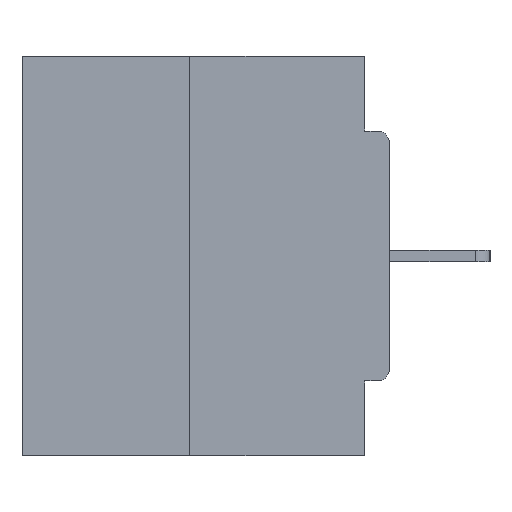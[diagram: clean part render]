
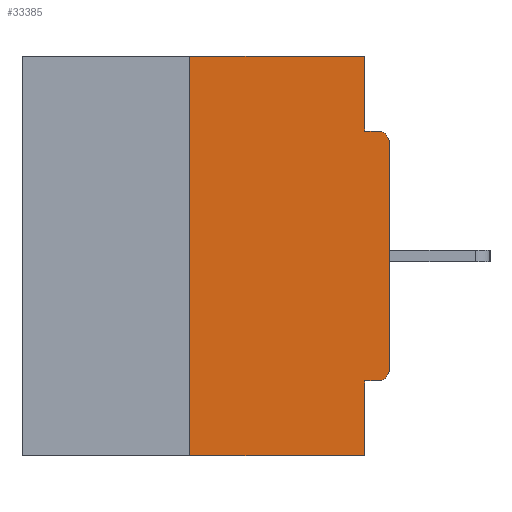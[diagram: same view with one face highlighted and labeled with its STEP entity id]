
A CAD part, left-side view. The second image highlights one B-rep face of the part: STEP entity #33385.
In plain terms, the highlighted planar face has unit normal (-1, 0, 0).
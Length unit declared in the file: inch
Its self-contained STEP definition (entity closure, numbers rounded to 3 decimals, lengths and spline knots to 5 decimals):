
#1274 = VERTEX_POINT ( 'NONE', #31369 ) ;
#2604 = CARTESIAN_POINT ( 'NONE',  ( 0., 0., -0.0935 ) ) ;
#3600 = AXIS2_PLACEMENT_3D ( 'NONE', #32483, #29717, #26374 ) ;
#3824 = VERTEX_POINT ( 'NONE', #5330 ) ;
#4188 = AXIS2_PLACEMENT_3D ( 'NONE', #30017, #5904, #33149 ) ;
#5330 = CARTESIAN_POINT ( 'NONE',  ( 0., 0.031, -0.4065 ) ) ;
#5664 = VECTOR ( 'NONE', #18033, 39.37008 ) ;
#5861 = CARTESIAN_POINT ( 'NONE',  ( 0., 0., -0.3915 ) ) ;
#5904 = DIRECTION ( 'NONE',  ( -1., 0., 0. ) ) ;
#6030 = ORIENTED_EDGE ( 'NONE', *, *, #16858, .F. ) ;
#6788 = CARTESIAN_POINT ( 'NONE',  ( 0., 0.031, -0.5 ) ) ;
#7313 = DIRECTION ( 'NONE',  ( 0., -1., 0. ) ) ;
#7596 = CARTESIAN_POINT ( 'NONE',  ( 0., 0.46, -0.5 ) ) ;
#7690 = DIRECTION ( 'NONE',  ( 0., 0., -1. ) ) ;
#7741 = AXIS2_PLACEMENT_3D ( 'NONE', #16851, #10987, #31230 ) ;
#10088 = VERTEX_POINT ( 'NONE', #12176 ) ;
#10491 = CARTESIAN_POINT ( 'NONE',  ( 0., 0.015, -0.0935 ) ) ;
#10602 = VERTEX_POINT ( 'NONE', #5861 ) ;
#10753 = DIRECTION ( 'NONE',  ( 0., 1., 0. ) ) ;
#10987 = DIRECTION ( 'NONE',  ( 1., 0., 0. ) ) ;
#11127 = EDGE_CURVE ( 'NONE', #16097, #1274, #31226, .T. ) ;
#11140 = CIRCLE ( 'NONE', #3600, 0.015 ) ;
#12176 = CARTESIAN_POINT ( 'NONE',  ( 0., 0.25, 0. ) ) ;
#13033 = DIRECTION ( 'NONE',  ( 0., 0., 1. ) ) ;
#13293 = CARTESIAN_POINT ( 'NONE',  ( 0., 0.015, -0.4065 ) ) ;
#13411 = VECTOR ( 'NONE', #29967, 39.37008 ) ;
#13440 = CARTESIAN_POINT ( 'NONE',  ( 0., 0., -0.1085 ) ) ;
#15806 = ORIENTED_EDGE ( 'NONE', *, *, #22872, .T. ) ;
#16097 = VERTEX_POINT ( 'NONE', #23859 ) ;
#16159 = LINE ( 'NONE', #19076, #30032 ) ;
#16303 = VERTEX_POINT ( 'NONE', #6788 ) ;
#16851 = CARTESIAN_POINT ( 'NONE',  ( 0., 0.46, 0. ) ) ;
#16858 = EDGE_CURVE ( 'NONE', #10088, #16097, #27702, .T. ) ;
#17041 = PLANE ( 'NONE',  #7741 ) ;
#17614 = CARTESIAN_POINT ( 'NONE',  ( 0., 0.031, -0.5 ) ) ;
#18033 = DIRECTION ( 'NONE',  ( 0., -1., 0. ) ) ;
#18091 = VECTOR ( 'NONE', #7690, 39.37008 ) ;
#19032 = VECTOR ( 'NONE', #10753, 39.37008 ) ;
#19076 = CARTESIAN_POINT ( 'NONE',  ( 0., 0.25, 0. ) ) ;
#19533 = DIRECTION ( 'NONE',  ( 0., -1., 0. ) ) ;
#19985 = EDGE_CURVE ( 'NONE', #21564, #10088, #16159, .T. ) ;
#20447 = ORIENTED_EDGE ( 'NONE', *, *, #33771, .F. ) ;
#21071 = CIRCLE ( 'NONE', #4188, 0.015 ) ;
#21079 = DIRECTION ( 'NONE',  ( 0., 0., 1. ) ) ;
#21564 = VERTEX_POINT ( 'NONE', #36127 ) ;
#21653 = EDGE_LOOP ( 'NONE', ( #6030, #34136, #28390, #24570, #20447, #22272, #15806, #34123, #37435, #36820 ) ) ;
#21986 = EDGE_CURVE ( 'NONE', #1274, #31187, #38257, .T. ) ;
#22272 = ORIENTED_EDGE ( 'NONE', *, *, #38462, .T. ) ;
#22681 = EDGE_CURVE ( 'NONE', #21564, #16303, #34457, .T. ) ;
#22765 = CARTESIAN_POINT ( 'NONE',  ( 0., 0.031, 0. ) ) ;
#22872 = EDGE_CURVE ( 'NONE', #10602, #31143, #24021, .T. ) ;
#23245 = VECTOR ( 'NONE', #21079, 39.37008 ) ;
#23859 = CARTESIAN_POINT ( 'NONE',  ( 0., 0.031, 0. ) ) ;
#24021 = LINE ( 'NONE', #27543, #23245 ) ;
#24570 = ORIENTED_EDGE ( 'NONE', *, *, #32243, .F. ) ;
#24749 = CARTESIAN_POINT ( 'NONE',  ( 0., 0.46, 0. ) ) ;
#26374 = DIRECTION ( 'NONE',  ( 0., 0., -1. ) ) ;
#27543 = CARTESIAN_POINT ( 'NONE',  ( 0., 0., 0. ) ) ;
#27702 = LINE ( 'NONE', #24749, #35041 ) ;
#28311 = VERTEX_POINT ( 'NONE', #13293 ) ;
#28390 = ORIENTED_EDGE ( 'NONE', *, *, #22681, .T. ) ;
#29396 = FACE_OUTER_BOUND ( 'NONE', #21653, .T. ) ;
#29717 = DIRECTION ( 'NONE',  ( -1., 0., 0. ) ) ;
#29967 = DIRECTION ( 'NONE',  ( 0., 0., -1. ) ) ;
#30017 = CARTESIAN_POINT ( 'NONE',  ( 0., 0.015, -0.1085 ) ) ;
#30032 = VECTOR ( 'NONE', #13033, 39.37008 ) ;
#31143 = VERTEX_POINT ( 'NONE', #13440 ) ;
#31187 = VERTEX_POINT ( 'NONE', #10491 ) ;
#31226 = LINE ( 'NONE', #22765, #18091 ) ;
#31230 = DIRECTION ( 'NONE',  ( 0., 0., -1. ) ) ;
#31369 = CARTESIAN_POINT ( 'NONE',  ( 0., 0.031, -0.0935 ) ) ;
#32243 = EDGE_CURVE ( 'NONE', #3824, #16303, #35663, .T. ) ;
#32483 = CARTESIAN_POINT ( 'NONE',  ( 0., 0.015, -0.3915 ) ) ;
#32611 = VECTOR ( 'NONE', #19533, 39.37008 ) ;
#33149 = DIRECTION ( 'NONE',  ( 0., 0., -1. ) ) ;
#33385 = ADVANCED_FACE ( 'NONE', ( #29396 ), #17041, .F. ) ;
#33771 = EDGE_CURVE ( 'NONE', #28311, #3824, #36805, .T. ) ;
#34123 = ORIENTED_EDGE ( 'NONE', *, *, #37679, .T. ) ;
#34136 = ORIENTED_EDGE ( 'NONE', *, *, #19985, .F. ) ;
#34457 = LINE ( 'NONE', #7596, #32611 ) ;
#35041 = VECTOR ( 'NONE', #7313, 39.37008 ) ;
#35663 = LINE ( 'NONE', #17614, #13411 ) ;
#36127 = CARTESIAN_POINT ( 'NONE',  ( 0., 0.25, -0.5 ) ) ;
#36608 = CARTESIAN_POINT ( 'NONE',  ( 0., 0., -0.4065 ) ) ;
#36805 = LINE ( 'NONE', #36608, #19032 ) ;
#36820 = ORIENTED_EDGE ( 'NONE', *, *, #11127, .F. ) ;
#37435 = ORIENTED_EDGE ( 'NONE', *, *, #21986, .F. ) ;
#37679 = EDGE_CURVE ( 'NONE', #31143, #31187, #21071, .T. ) ;
#38257 = LINE ( 'NONE', #2604, #5664 ) ;
#38462 = EDGE_CURVE ( 'NONE', #28311, #10602, #11140, .T. ) ;
